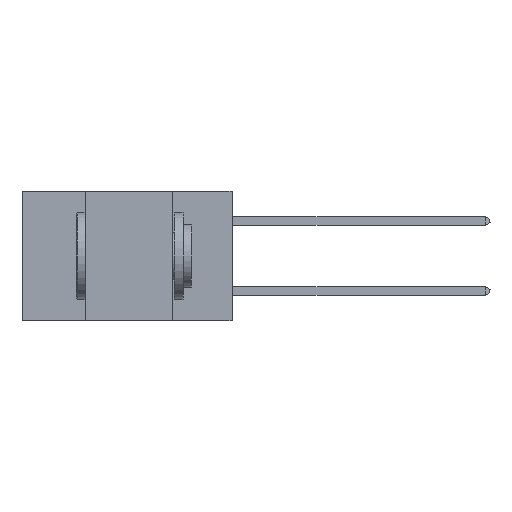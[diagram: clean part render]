
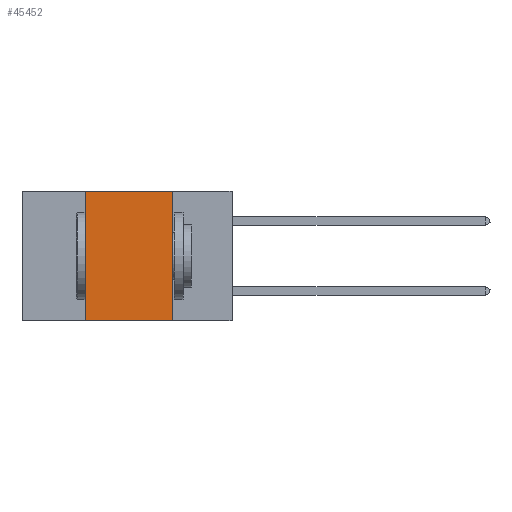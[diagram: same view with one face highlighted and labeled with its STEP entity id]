
A CAD part, left-side view. The second image highlights one B-rep face of the part: STEP entity #45452.
In plain terms, the highlighted planar face has unit normal (-1, 0, 0).
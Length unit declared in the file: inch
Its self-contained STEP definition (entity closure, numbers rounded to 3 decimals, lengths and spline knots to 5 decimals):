
#2853 = LINE ( 'NONE', #38979, #38999 ) ;
#3067 = LINE ( 'NONE', #28053, #21178 ) ;
#3244 = VECTOR ( 'NONE', #21333, 39.37008 ) ;
#3315 = EDGE_CURVE ( 'NONE', #14043, #33544, #19630, .T. ) ;
#4745 = CARTESIAN_POINT ( 'NONE',  ( 0., 0.6, 0. ) ) ;
#5137 = VECTOR ( 'NONE', #27213, 39.37008 ) ;
#6392 = CARTESIAN_POINT ( 'NONE',  ( 0., 0.17, -0.37 ) ) ;
#9871 = FACE_OUTER_BOUND ( 'NONE', #15859, .T. ) ;
#10955 = ORIENTED_EDGE ( 'NONE', *, *, #3315, .T. ) ;
#14041 = DIRECTION ( 'NONE',  ( 0., -1., 0. ) ) ;
#14043 = VERTEX_POINT ( 'NONE', #33836 ) ;
#15859 = EDGE_LOOP ( 'NONE', ( #31940, #34308, #17862, #10955 ) ) ;
#17411 = CARTESIAN_POINT ( 'NONE',  ( 0., 0.42, 0. ) ) ;
#17627 = DIRECTION ( 'NONE',  ( 0., 0., 1. ) ) ;
#17862 = ORIENTED_EDGE ( 'NONE', *, *, #33493, .F. ) ;
#19630 = LINE ( 'NONE', #39144, #3244 ) ;
#21178 = VECTOR ( 'NONE', #17627, 39.37008 ) ;
#21333 = DIRECTION ( 'NONE',  ( 0., -1., 0. ) ) ;
#24664 = EDGE_CURVE ( 'NONE', #45886, #33544, #39633, .T. ) ;
#25402 = CARTESIAN_POINT ( 'NONE',  ( 0., 0.17, 0. ) ) ;
#26833 = DIRECTION ( 'NONE',  ( 0., 0., -1. ) ) ;
#27213 = DIRECTION ( 'NONE',  ( 0., 0., -1. ) ) ;
#28053 = CARTESIAN_POINT ( 'NONE',  ( 0., 0.42, 0. ) ) ;
#31940 = ORIENTED_EDGE ( 'NONE', *, *, #24664, .F. ) ;
#33493 = EDGE_CURVE ( 'NONE', #14043, #43058, #3067, .T. ) ;
#33544 = VERTEX_POINT ( 'NONE', #6392 ) ;
#33836 = CARTESIAN_POINT ( 'NONE',  ( 0., 0.42, -0.37 ) ) ;
#34264 = PLANE ( 'NONE',  #42317 ) ;
#34308 = ORIENTED_EDGE ( 'NONE', *, *, #42556, .F. ) ;
#37900 = DIRECTION ( 'NONE',  ( 1., 0., 0. ) ) ;
#38407 = CARTESIAN_POINT ( 'NONE',  ( 0., 0.17, 0. ) ) ;
#38979 = CARTESIAN_POINT ( 'NONE',  ( 0., 0.6, 0. ) ) ;
#38999 = VECTOR ( 'NONE', #14041, 39.37008 ) ;
#39144 = CARTESIAN_POINT ( 'NONE',  ( 0., 0.6, -0.37 ) ) ;
#39633 = LINE ( 'NONE', #38407, #5137 ) ;
#42317 = AXIS2_PLACEMENT_3D ( 'NONE', #4745, #37900, #26833 ) ;
#42556 = EDGE_CURVE ( 'NONE', #43058, #45886, #2853, .T. ) ;
#43058 = VERTEX_POINT ( 'NONE', #17411 ) ;
#45452 = ADVANCED_FACE ( 'NONE', ( #9871 ), #34264, .F. ) ;
#45886 = VERTEX_POINT ( 'NONE', #25402 ) ;
